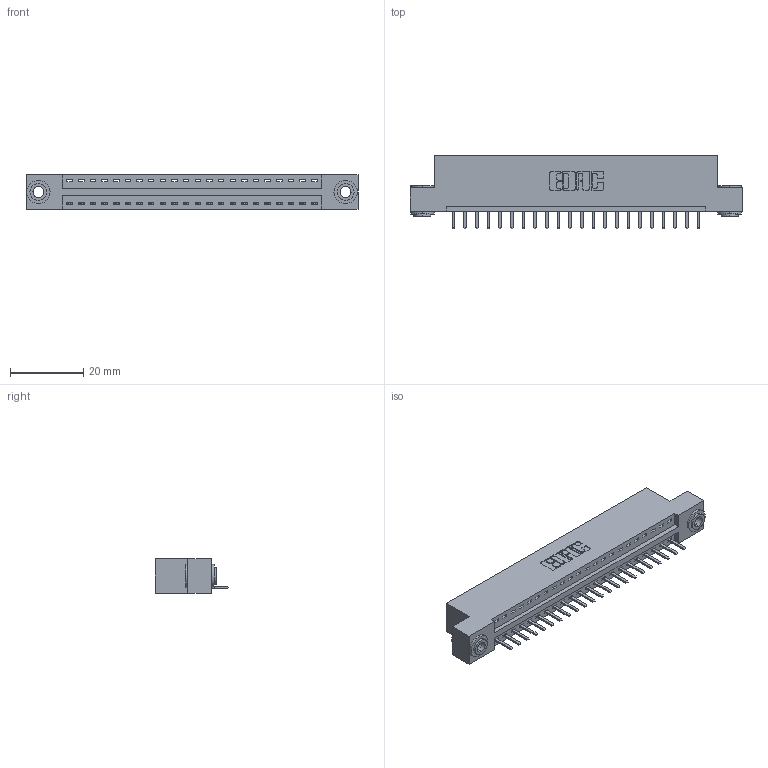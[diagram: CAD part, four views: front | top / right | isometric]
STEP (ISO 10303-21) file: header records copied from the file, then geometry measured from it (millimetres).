
FILE_DESCRIPTION (( 'STEP AP203' ), '1' );
FILE_NAME ('396-022-520-103.STEP', '2018-09-01T08:24:26', ( '' ), ( '' ), 'SwSTEP 2.0', 'SolidWorks 2016', '' );
FILE_SCHEMA (( 'CONFIG_CONTROL_DESIGN' ));
Length unit declared in the file: inch
Products named in the file (4): 396-022-520-103; 346 Part_Flush Mounting Lugs - 0.156 Dia-TH; 345-292-001_345-293-120; 345-250-002_345-250-002-102
Assembly tree (25 placements, depth 2):
  396-022-520-103
    346 Part_Flush Mounting Lugs - 0.156 Dia-TH
    345-292-001_345-293-120  x22
    345-250-002_345-250-002-102  x2
Bounding box: 90.42 x 20.02 x 9.4 mm (x, y, z)
Volume: 8473.9 mm3; surface area: 10383.4 mm2
Topology: 25 solids, 25 shells, 1524 faces, 4453 edges, 2906 vertices
Faces by surface type: plane 1010, cylinder 506, cone 8
Entity records: 17110 total; most frequent: CARTESIAN_POINT 2929, ORIENTED_EDGE 2866, DIRECTION 2627, EDGE_CURVE 1433, VECTOR 1185, LINE 1185, VERTEX_POINT 950, AXIS2_PLACEMENT_3D 721
